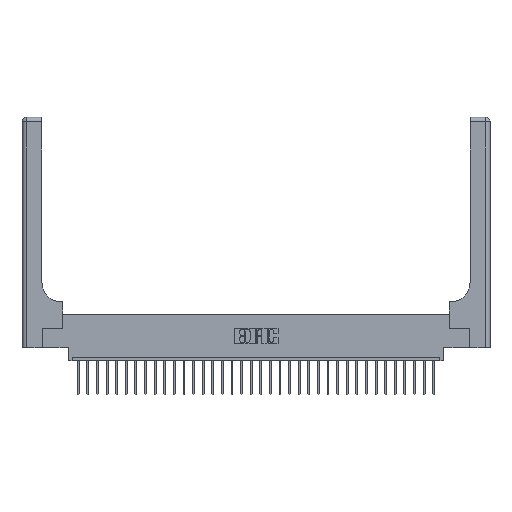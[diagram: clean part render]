
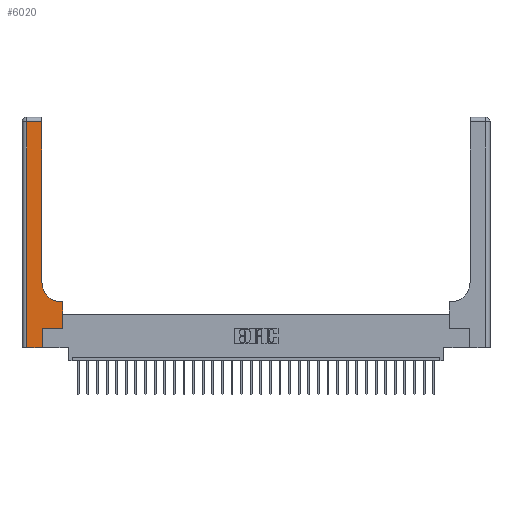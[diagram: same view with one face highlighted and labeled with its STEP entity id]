
A CAD part, top view. The second image highlights one B-rep face of the part: STEP entity #6020.
In plain terms, the highlighted planar face has unit normal (0, 0, 1).
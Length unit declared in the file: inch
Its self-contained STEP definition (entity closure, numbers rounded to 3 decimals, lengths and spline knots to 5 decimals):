
#469 = EDGE_LOOP ( 'NONE', ( #20519, #7632, #16712, #14341, #11206, #26275, #26694, #7806, #17454 ) ) ;
#1070 = LINE ( 'NONE', #16806, #14666 ) ;
#1325 = VERTEX_POINT ( 'NONE', #7214 ) ;
#1863 = VERTEX_POINT ( 'NONE', #3827 ) ;
#1865 = DIRECTION ( 'NONE',  ( 1., 0., 0. ) ) ;
#2025 = CARTESIAN_POINT ( 'NONE',  ( 0.265, 0., 0.37 ) ) ;
#2883 = CARTESIAN_POINT ( 'NONE',  ( 0.51, 0.85, 0.37 ) ) ;
#3027 = DIRECTION ( 'NONE',  ( 1., 0., 0. ) ) ;
#3233 = CARTESIAN_POINT ( 'NONE',  ( 0.26, 0.6, 0.37 ) ) ;
#3438 = CARTESIAN_POINT ( 'NONE',  ( 0., 0., 0.37 ) ) ;
#3576 = LINE ( 'NONE', #3438, #15724 ) ;
#3827 = CARTESIAN_POINT ( 'NONE',  ( 0.528, 0.6, 0.37 ) ) ;
#3884 = AXIS2_PLACEMENT_3D ( 'NONE', #8114, #14776, #12802 ) ;
#6020 = ADVANCED_FACE ( 'NONE', ( #26454 ), #10396, .F. ) ;
#6238 = LINE ( 'NONE', #22428, #20789 ) ;
#6369 = EDGE_CURVE ( 'NONE', #21609, #1325, #6238, .T. ) ;
#6464 = VECTOR ( 'NONE', #20027, 39.37008 ) ;
#6499 = EDGE_CURVE ( 'NONE', #18151, #21609, #22898, .T. ) ;
#7214 = CARTESIAN_POINT ( 'NONE',  ( 0.528, 0.25, 0.37 ) ) ;
#7467 = DIRECTION ( 'NONE',  ( -1., 0., 0. ) ) ;
#7632 = ORIENTED_EDGE ( 'NONE', *, *, #17473, .T. ) ;
#7776 = CIRCLE ( 'NONE', #9234, 0.25 ) ;
#7806 = ORIENTED_EDGE ( 'NONE', *, *, #27848, .T. ) ;
#7901 = CARTESIAN_POINT ( 'NONE',  ( 0., 2.94, 0.37 ) ) ;
#8114 = CARTESIAN_POINT ( 'NONE',  ( 0., 3., 0.37 ) ) ;
#9234 = AXIS2_PLACEMENT_3D ( 'NONE', #2883, #9540, #3027 ) ;
#9540 = DIRECTION ( 'NONE',  ( 0., 0., -1. ) ) ;
#9543 = VERTEX_POINT ( 'NONE', #24099 ) ;
#10396 = PLANE ( 'NONE',  #3884 ) ;
#10791 = CARTESIAN_POINT ( 'NONE',  ( 0.06, 0., 0.37 ) ) ;
#10813 = CARTESIAN_POINT ( 'NONE',  ( 0.528, 0.25, 0.37 ) ) ;
#11081 = VECTOR ( 'NONE', #7467, 39.37008 ) ;
#11206 = ORIENTED_EDGE ( 'NONE', *, *, #6499, .T. ) ;
#12802 = DIRECTION ( 'NONE',  ( -1., 0., 0. ) ) ;
#12908 = EDGE_CURVE ( 'NONE', #13876, #28569, #21233, .T. ) ;
#13339 = EDGE_CURVE ( 'NONE', #9543, #13876, #7776, .T. ) ;
#13876 = VERTEX_POINT ( 'NONE', #20770 ) ;
#14341 = ORIENTED_EDGE ( 'NONE', *, *, #22112, .T. ) ;
#14412 = LINE ( 'NONE', #7901, #15660 ) ;
#14429 = LINE ( 'NONE', #3233, #11081 ) ;
#14516 = VECTOR ( 'NONE', #21962, 39.37008 ) ;
#14661 = DIRECTION ( 'NONE',  ( 0., -1., 0. ) ) ;
#14666 = VECTOR ( 'NONE', #14661, 39.37008 ) ;
#14776 = DIRECTION ( 'NONE',  ( 0., 0., -1. ) ) ;
#15660 = VECTOR ( 'NONE', #26097, 39.37008 ) ;
#15724 = VECTOR ( 'NONE', #24041, 39.37008 ) ;
#16712 = ORIENTED_EDGE ( 'NONE', *, *, #18709, .T. ) ;
#16806 = CARTESIAN_POINT ( 'NONE',  ( 0.06, 3., 0.37 ) ) ;
#17302 = EDGE_CURVE ( 'NONE', #1325, #1863, #24590, .T. ) ;
#17454 = ORIENTED_EDGE ( 'NONE', *, *, #13339, .T. ) ;
#17473 = EDGE_CURVE ( 'NONE', #28569, #22276, #14412, .T. ) ;
#17906 = VECTOR ( 'NONE', #25485, 39.37008 ) ;
#18151 = VERTEX_POINT ( 'NONE', #29281 ) ;
#18319 = CARTESIAN_POINT ( 'NONE',  ( 0.26, 2.94, 0.37 ) ) ;
#18709 = EDGE_CURVE ( 'NONE', #22276, #26698, #1070, .T. ) ;
#19374 = CARTESIAN_POINT ( 'NONE',  ( 0.265, 0.25, 0.37 ) ) ;
#19395 = CARTESIAN_POINT ( 'NONE',  ( 0.26, 3., 0.37 ) ) ;
#20027 = DIRECTION ( 'NONE',  ( 0., 1., 0. ) ) ;
#20519 = ORIENTED_EDGE ( 'NONE', *, *, #12908, .T. ) ;
#20770 = CARTESIAN_POINT ( 'NONE',  ( 0.26, 0.85, 0.37 ) ) ;
#20789 = VECTOR ( 'NONE', #1865, 39.37008 ) ;
#21233 = LINE ( 'NONE', #19395, #14516 ) ;
#21609 = VERTEX_POINT ( 'NONE', #19374 ) ;
#21962 = DIRECTION ( 'NONE',  ( 0., 1., 0. ) ) ;
#22112 = EDGE_CURVE ( 'NONE', #26698, #18151, #3576, .T. ) ;
#22276 = VERTEX_POINT ( 'NONE', #22808 ) ;
#22428 = CARTESIAN_POINT ( 'NONE',  ( 0.265, 0.25, 0.37 ) ) ;
#22808 = CARTESIAN_POINT ( 'NONE',  ( 0.06, 2.94, 0.37 ) ) ;
#22898 = LINE ( 'NONE', #2025, #17906 ) ;
#24041 = DIRECTION ( 'NONE',  ( 1., 0., 0. ) ) ;
#24099 = CARTESIAN_POINT ( 'NONE',  ( 0.51, 0.6, 0.37 ) ) ;
#24590 = LINE ( 'NONE', #10813, #6464 ) ;
#25485 = DIRECTION ( 'NONE',  ( 0., 1., 0. ) ) ;
#26097 = DIRECTION ( 'NONE',  ( -1., 0., 0. ) ) ;
#26275 = ORIENTED_EDGE ( 'NONE', *, *, #6369, .T. ) ;
#26454 = FACE_OUTER_BOUND ( 'NONE', #469, .T. ) ;
#26694 = ORIENTED_EDGE ( 'NONE', *, *, #17302, .T. ) ;
#26698 = VERTEX_POINT ( 'NONE', #10791 ) ;
#27848 = EDGE_CURVE ( 'NONE', #1863, #9543, #14429, .T. ) ;
#28569 = VERTEX_POINT ( 'NONE', #18319 ) ;
#29281 = CARTESIAN_POINT ( 'NONE',  ( 0.265, 0., 0.37 ) ) ;
